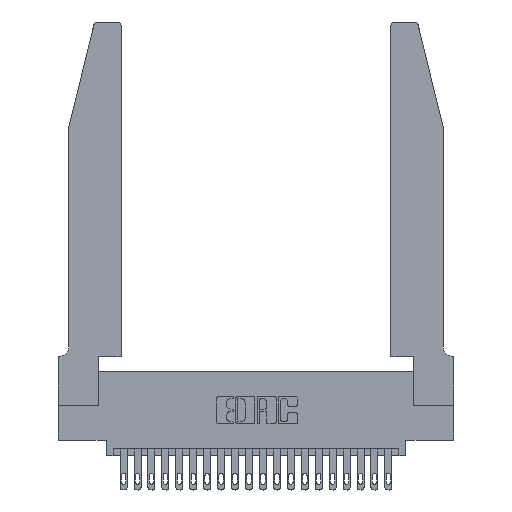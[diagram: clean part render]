
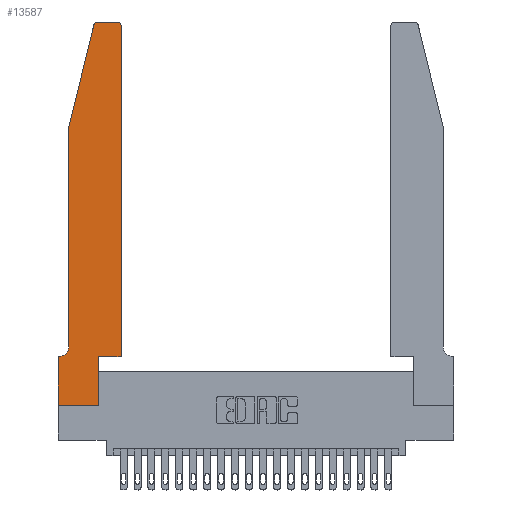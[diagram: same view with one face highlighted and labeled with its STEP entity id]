
A CAD part, top view. The second image highlights one B-rep face of the part: STEP entity #13587.
In plain terms, the highlighted planar face has unit normal (0, 0, 1).
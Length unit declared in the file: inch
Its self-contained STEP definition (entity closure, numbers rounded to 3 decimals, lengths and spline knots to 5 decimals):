
#122 = VECTOR ( 'NONE', #9444, 39.37008 ) ;
#202 = ORIENTED_EDGE ( 'NONE', *, *, #2357, .T. ) ;
#430 = LINE ( 'NONE', #2530, #11179 ) ;
#696 = VERTEX_POINT ( 'NONE', #15642 ) ;
#902 = CARTESIAN_POINT ( 'NONE',  ( 0.25487, 2.72718, 0.37 ) ) ;
#996 = CARTESIAN_POINT ( 'NONE',  ( 0.4205, 2.72, 0.37 ) ) ;
#1196 = LINE ( 'NONE', #8479, #23338 ) ;
#1271 = EDGE_LOOP ( 'NONE', ( #17834, #3977, #4544, #202, #4078, #21376, #3424, #5559, #22873, #9371, #14151, #14346 ) ) ;
#1291 = CARTESIAN_POINT ( 'NONE',  ( 0., 0.35, 0.37 ) ) ;
#1306 = EDGE_CURVE ( 'NONE', #10468, #14630, #4048, .T. ) ;
#1341 = EDGE_CURVE ( 'NONE', #2012, #11895, #10282, .T. ) ;
#1503 = VECTOR ( 'NONE', #5839, 39.37008 ) ;
#1587 = EDGE_CURVE ( 'NONE', #4472, #21099, #12001, .T. ) ;
#2012 = VERTEX_POINT ( 'NONE', #17781 ) ;
#2357 = EDGE_CURVE ( 'NONE', #21110, #10468, #20745, .T. ) ;
#2530 = CARTESIAN_POINT ( 'NONE',  ( 0., 0., 0.37 ) ) ;
#3054 = DIRECTION ( 'NONE',  ( -1., 0., 0. ) ) ;
#3424 = ORIENTED_EDGE ( 'NONE', *, *, #13878, .T. ) ;
#3977 = ORIENTED_EDGE ( 'NONE', *, *, #1587, .T. ) ;
#4048 = CIRCLE ( 'NONE', #12717, 0.07 ) ;
#4078 = ORIENTED_EDGE ( 'NONE', *, *, #1306, .T. ) ;
#4472 = VERTEX_POINT ( 'NONE', #5746 ) ;
#4544 = ORIENTED_EDGE ( 'NONE', *, *, #17809, .T. ) ;
#4740 = DIRECTION ( 'NONE',  ( -0.239, -0.971, 0. ) ) ;
#4891 = DIRECTION ( 'NONE',  ( 1., 0., 0. ) ) ;
#5057 = DIRECTION ( 'NONE',  ( 0., 0., 1. ) ) ;
#5452 = VECTOR ( 'NONE', #9732, 39.37008 ) ;
#5559 = ORIENTED_EDGE ( 'NONE', *, *, #12739, .T. ) ;
#5746 = CARTESIAN_POINT ( 'NONE',  ( 0.284, 2.75, 0.37 ) ) ;
#5839 = DIRECTION ( 'NONE',  ( 0., -1., 0. ) ) ;
#6141 = AXIS2_PLACEMENT_3D ( 'NONE', #996, #8415, #10224 ) ;
#6591 = DIRECTION ( 'NONE',  ( -1., 0., 0. ) ) ;
#6688 = EDGE_CURVE ( 'NONE', #9293, #2012, #7313, .T. ) ;
#7313 = LINE ( 'NONE', #13633, #11298 ) ;
#7419 = VECTOR ( 'NONE', #23144, 39.37008 ) ;
#7532 = CARTESIAN_POINT ( 'NONE',  ( 0.0055, 0.35, 0.37 ) ) ;
#7966 = CARTESIAN_POINT ( 'NONE',  ( 0.4505, 0.35, 0.37 ) ) ;
#8299 = FACE_OUTER_BOUND ( 'NONE', #1271, .T. ) ;
#8415 = DIRECTION ( 'NONE',  ( 0., 0., 1. ) ) ;
#8479 = CARTESIAN_POINT ( 'NONE',  ( 0.0755, 2., 0.37 ) ) ;
#9136 = EDGE_CURVE ( 'NONE', #11895, #696, #20078, .T. ) ;
#9293 = VERTEX_POINT ( 'NONE', #15809 ) ;
#9371 = ORIENTED_EDGE ( 'NONE', *, *, #1341, .T. ) ;
#9398 = CARTESIAN_POINT ( 'NONE',  ( 0.0755, 0.42, 0.37 ) ) ;
#9444 = DIRECTION ( 'NONE',  ( -1., 0., 0. ) ) ;
#9507 = EDGE_CURVE ( 'NONE', #696, #13780, #10581, .T. ) ;
#9732 = DIRECTION ( 'NONE',  ( 1., 0., 0. ) ) ;
#10224 = DIRECTION ( 'NONE',  ( 1., 0., 0. ) ) ;
#10282 = LINE ( 'NONE', #10638, #5452 ) ;
#10295 = DIRECTION ( 'NONE',  ( 0., 1., 0. ) ) ;
#10413 = CARTESIAN_POINT ( 'NONE',  ( 0.0755, 0.35, 0.37 ) ) ;
#10468 = VERTEX_POINT ( 'NONE', #9398 ) ;
#10525 = CARTESIAN_POINT ( 'NONE',  ( 0., 0.35, 0.37 ) ) ;
#10581 = CIRCLE ( 'NONE', #6141, 0.03 ) ;
#10638 = CARTESIAN_POINT ( 'NONE',  ( 0.4505, 0.35, 0.37 ) ) ;
#11179 = VECTOR ( 'NONE', #15195, 39.37008 ) ;
#11298 = VECTOR ( 'NONE', #19267, 39.37008 ) ;
#11895 = VERTEX_POINT ( 'NONE', #7966 ) ;
#12001 = CIRCLE ( 'NONE', #18643, 0.03 ) ;
#12380 = DIRECTION ( 'NONE',  ( 1., 0., 0. ) ) ;
#12585 = CARTESIAN_POINT ( 'NONE',  ( 0.2605, 2.75, 0.37 ) ) ;
#12717 = AXIS2_PLACEMENT_3D ( 'NONE', #23422, #14149, #3054 ) ;
#12739 = EDGE_CURVE ( 'NONE', #21017, #9293, #430, .T. ) ;
#12789 = LINE ( 'NONE', #10413, #15063 ) ;
#13587 = ADVANCED_FACE ( 'NONE', ( #8299 ), #23017, .T. ) ;
#13633 = CARTESIAN_POINT ( 'NONE',  ( 0.2865, 0.35, 0.37 ) ) ;
#13780 = VERTEX_POINT ( 'NONE', #16765 ) ;
#13878 = EDGE_CURVE ( 'NONE', #21260, #21017, #14805, .T. ) ;
#13947 = DIRECTION ( 'NONE',  ( 0., 0., 1. ) ) ;
#14149 = DIRECTION ( 'NONE',  ( 0., 0., -1. ) ) ;
#14151 = ORIENTED_EDGE ( 'NONE', *, *, #9136, .T. ) ;
#14211 = CARTESIAN_POINT ( 'NONE',  ( 0.284, 2.72, 0.37 ) ) ;
#14346 = ORIENTED_EDGE ( 'NONE', *, *, #9507, .T. ) ;
#14630 = VERTEX_POINT ( 'NONE', #7532 ) ;
#14805 = LINE ( 'NONE', #17914, #7419 ) ;
#14820 = EDGE_CURVE ( 'NONE', #14630, #21260, #12789, .T. ) ;
#15063 = VECTOR ( 'NONE', #6591, 39.37008 ) ;
#15195 = DIRECTION ( 'NONE',  ( 1., 0., 0. ) ) ;
#15642 = CARTESIAN_POINT ( 'NONE',  ( 0.4505, 2.72, 0.37 ) ) ;
#15809 = CARTESIAN_POINT ( 'NONE',  ( 0.2865, 0., 0.37 ) ) ;
#16491 = EDGE_CURVE ( 'NONE', #13780, #4472, #18815, .T. ) ;
#16765 = CARTESIAN_POINT ( 'NONE',  ( 0.4205, 2.75, 0.37 ) ) ;
#16959 = CARTESIAN_POINT ( 'NONE',  ( 0., 0., 0.37 ) ) ;
#17781 = CARTESIAN_POINT ( 'NONE',  ( 0.2865, 0.35, 0.37 ) ) ;
#17809 = EDGE_CURVE ( 'NONE', #21099, #21110, #1196, .T. ) ;
#17834 = ORIENTED_EDGE ( 'NONE', *, *, #16491, .T. ) ;
#17914 = CARTESIAN_POINT ( 'NONE',  ( 0., 0., 0.37 ) ) ;
#18142 = AXIS2_PLACEMENT_3D ( 'NONE', #1291, #13947, #4891 ) ;
#18643 = AXIS2_PLACEMENT_3D ( 'NONE', #14211, #5057, #12380 ) ;
#18700 = CARTESIAN_POINT ( 'NONE',  ( 0.0755, 2., 0.37 ) ) ;
#18815 = LINE ( 'NONE', #12585, #122 ) ;
#19267 = DIRECTION ( 'NONE',  ( 0., 1., 0. ) ) ;
#19420 = CARTESIAN_POINT ( 'NONE',  ( 0.4505, 0.35, 0.37 ) ) ;
#20078 = LINE ( 'NONE', #19420, #20375 ) ;
#20375 = VECTOR ( 'NONE', #10295, 39.37008 ) ;
#20745 = LINE ( 'NONE', #22466, #1503 ) ;
#21017 = VERTEX_POINT ( 'NONE', #16959 ) ;
#21099 = VERTEX_POINT ( 'NONE', #902 ) ;
#21110 = VERTEX_POINT ( 'NONE', #18700 ) ;
#21260 = VERTEX_POINT ( 'NONE', #10525 ) ;
#21376 = ORIENTED_EDGE ( 'NONE', *, *, #14820, .T. ) ;
#22466 = CARTESIAN_POINT ( 'NONE',  ( 0.0755, 2., 0.37 ) ) ;
#22873 = ORIENTED_EDGE ( 'NONE', *, *, #6688, .T. ) ;
#23017 = PLANE ( 'NONE',  #18142 ) ;
#23144 = DIRECTION ( 'NONE',  ( 0., -1., 0. ) ) ;
#23338 = VECTOR ( 'NONE', #4740, 39.37008 ) ;
#23422 = CARTESIAN_POINT ( 'NONE',  ( 0.0055, 0.42, 0.37 ) ) ;
